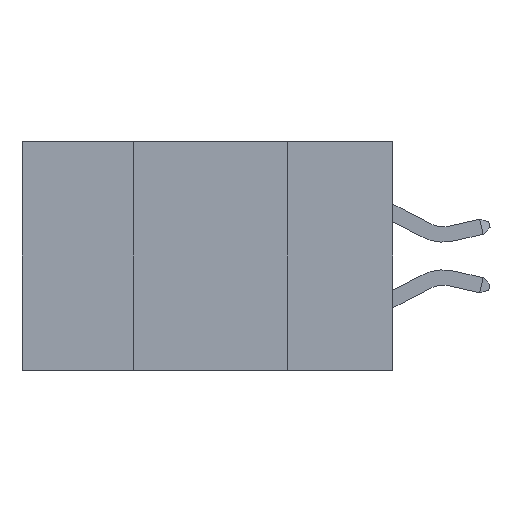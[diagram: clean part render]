
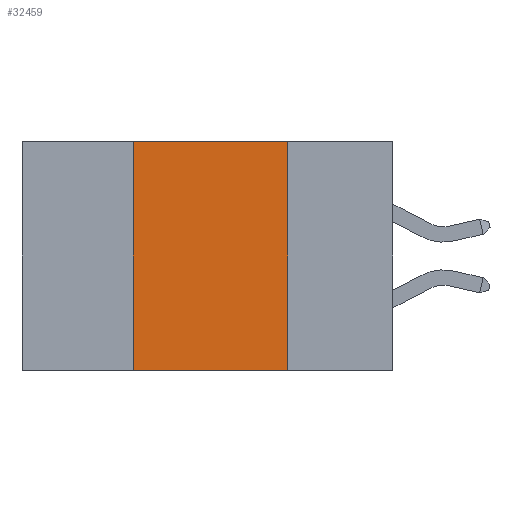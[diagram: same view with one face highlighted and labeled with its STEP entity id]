
A CAD part, left-side view. The second image highlights one B-rep face of the part: STEP entity #32459.
In plain terms, the highlighted planar face has unit normal (-1, 0, 0).
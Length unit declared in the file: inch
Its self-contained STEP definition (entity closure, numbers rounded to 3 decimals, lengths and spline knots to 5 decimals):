
#183 = VECTOR ( 'NONE', #4973, 39.37008 ) ;
#1870 = AXIS2_PLACEMENT_3D ( 'NONE', #11239, #21682, #23926 ) ;
#2323 = VERTEX_POINT ( 'NONE', #29792 ) ;
#3386 = VERTEX_POINT ( 'NONE', #23259 ) ;
#4441 = VERTEX_POINT ( 'NONE', #24328 ) ;
#4973 = DIRECTION ( 'NONE',  ( 0., -1., 0. ) ) ;
#5333 = CARTESIAN_POINT ( 'NONE',  ( 0., 0.17, 0. ) ) ;
#5601 = FACE_OUTER_BOUND ( 'NONE', #10790, .T. ) ;
#5716 = ORIENTED_EDGE ( 'NONE', *, *, #24169, .T. ) ;
#6932 = ORIENTED_EDGE ( 'NONE', *, *, #31834, .F. ) ;
#10790 = EDGE_LOOP ( 'NONE', ( #27018, #6932, #26611, #5716 ) ) ;
#11239 = CARTESIAN_POINT ( 'NONE',  ( 0., 0.6, 0. ) ) ;
#11320 = VERTEX_POINT ( 'NONE', #30307 ) ;
#11632 = DIRECTION ( 'NONE',  ( 0., 0., -1. ) ) ;
#12595 = EDGE_CURVE ( 'NONE', #11320, #4441, #16377, .T. ) ;
#12731 = CARTESIAN_POINT ( 'NONE',  ( 0., 0.6, -0.37 ) ) ;
#12864 = LINE ( 'NONE', #5333, #29185 ) ;
#13488 = PLANE ( 'NONE',  #1870 ) ;
#13791 = VECTOR ( 'NONE', #32086, 39.37008 ) ;
#16377 = LINE ( 'NONE', #31920, #13791 ) ;
#17119 = VECTOR ( 'NONE', #17192, 39.37008 ) ;
#17192 = DIRECTION ( 'NONE',  ( 0., -1., 0. ) ) ;
#21682 = DIRECTION ( 'NONE',  ( 1., 0., 0. ) ) ;
#22818 = LINE ( 'NONE', #12731, #17119 ) ;
#23259 = CARTESIAN_POINT ( 'NONE',  ( 0., 0.17, 0. ) ) ;
#23926 = DIRECTION ( 'NONE',  ( 0., 0., -1. ) ) ;
#24169 = EDGE_CURVE ( 'NONE', #11320, #2323, #22818, .T. ) ;
#24328 = CARTESIAN_POINT ( 'NONE',  ( 0., 0.42, 0. ) ) ;
#26016 = CARTESIAN_POINT ( 'NONE',  ( 0., 0.6, 0. ) ) ;
#26019 = EDGE_CURVE ( 'NONE', #3386, #2323, #12864, .T. ) ;
#26611 = ORIENTED_EDGE ( 'NONE', *, *, #12595, .F. ) ;
#27018 = ORIENTED_EDGE ( 'NONE', *, *, #26019, .F. ) ;
#29185 = VECTOR ( 'NONE', #11632, 39.37008 ) ;
#29792 = CARTESIAN_POINT ( 'NONE',  ( 0., 0.17, -0.37 ) ) ;
#30307 = CARTESIAN_POINT ( 'NONE',  ( 0., 0.42, -0.37 ) ) ;
#30785 = LINE ( 'NONE', #26016, #183 ) ;
#31834 = EDGE_CURVE ( 'NONE', #4441, #3386, #30785, .T. ) ;
#31920 = CARTESIAN_POINT ( 'NONE',  ( 0., 0.42, 0. ) ) ;
#32086 = DIRECTION ( 'NONE',  ( 0., 0., 1. ) ) ;
#32459 = ADVANCED_FACE ( 'NONE', ( #5601 ), #13488, .F. ) ;
